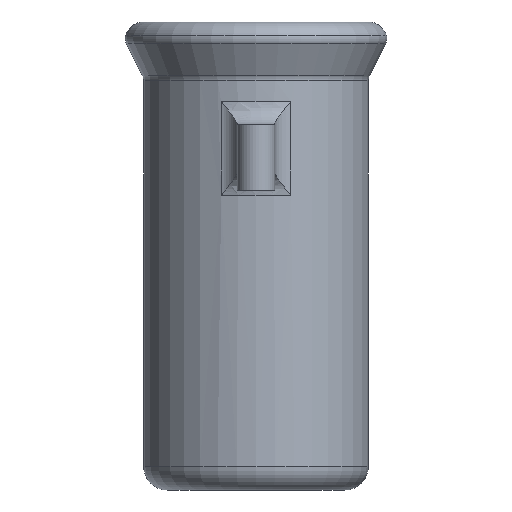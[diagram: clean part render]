
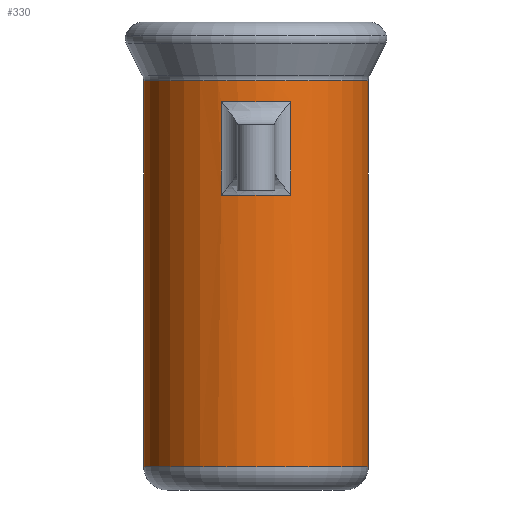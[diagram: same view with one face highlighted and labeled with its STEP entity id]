
A CAD part, front view. The second image highlights one B-rep face of the part: STEP entity #330.
In plain terms, the highlighted cylindrical face has radius 15.24 mm (diameter 30.48 mm), a partial arc.
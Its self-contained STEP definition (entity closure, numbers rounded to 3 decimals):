
#3 = EDGE_LOOP ( 'NONE', ( #1440, #1247, #1269, #567 ) ) ;
#60 = AXIS2_PLACEMENT_3D ( 'NONE', #1375, #1349, #1344 ) ;
#120 = FACE_OUTER_BOUND ( 'NONE', #3, .T. ) ;
#125 = LINE ( 'NONE', #1165, #603 ) ;
#192 = EDGE_CURVE ( 'NONE', #564, #1615, #839, .T. ) ;
#237 = CARTESIAN_POINT ( 'NONE',  ( 4.73, -14.488, 52.705 ) ) ;
#330 = ADVANCED_FACE ( 'NONE', ( #120, #961 ), #1234, .T. ) ;
#337 = DIRECTION ( 'NONE',  ( 1., 0., 0. ) ) ;
#349 = VECTOR ( 'NONE', #1202, 1000. ) ;
#352 = DIRECTION ( 'NONE',  ( 0., 0., 1. ) ) ;
#359 = CARTESIAN_POINT ( 'NONE',  ( 0., 0., 52.705 ) ) ;
#370 = CARTESIAN_POINT ( 'NONE',  ( -15.24, 0., 3.175 ) ) ;
#423 = VERTEX_POINT ( 'NONE', #1650 ) ;
#430 = VECTOR ( 'NONE', #542, 1000. ) ;
#456 = EDGE_CURVE ( 'NONE', #564, #423, #1716, .T. ) ;
#457 = ORIENTED_EDGE ( 'NONE', *, *, #522, .T. ) ;
#471 = EDGE_CURVE ( 'NONE', #1615, #534, #598, .T. ) ;
#475 = LINE ( 'NONE', #640, #430 ) ;
#498 = CARTESIAN_POINT ( 'NONE',  ( -4.73, -14.488, 40.005 ) ) ;
#500 = EDGE_CURVE ( 'NONE', #534, #423, #1430, .T. ) ;
#505 = EDGE_CURVE ( 'NONE', #1567, #708, #1121, .T. ) ;
#511 = DIRECTION ( 'NONE',  ( 1., 0., 0. ) ) ;
#514 = EDGE_CURVE ( 'NONE', #708, #1564, #475, .T. ) ;
#517 = EDGE_CURVE ( 'NONE', #1564, #570, #1556, .T. ) ;
#522 = EDGE_CURVE ( 'NONE', #570, #1567, #125, .T. ) ;
#525 = DIRECTION ( 'NONE',  ( 0., 0., -1. ) ) ;
#532 = CARTESIAN_POINT ( 'NONE',  ( 0., 0., 40.005 ) ) ;
#534 = VERTEX_POINT ( 'NONE', #370 ) ;
#542 = DIRECTION ( 'NONE',  ( 0., 0., 1. ) ) ;
#546 = DIRECTION ( 'NONE',  ( 1., 0., 0. ) ) ;
#553 = DIRECTION ( 'NONE',  ( 0., 0., 1. ) ) ;
#564 = VERTEX_POINT ( 'NONE', #1172 ) ;
#567 = ORIENTED_EDGE ( 'NONE', *, *, #500, .T. ) ;
#570 = VERTEX_POINT ( 'NONE', #237 ) ;
#598 = LINE ( 'NONE', #894, #349 ) ;
#603 = VECTOR ( 'NONE', #633, 1000. ) ;
#622 = CARTESIAN_POINT ( 'NONE',  ( 0., 0., 3.175 ) ) ;
#633 = DIRECTION ( 'NONE',  ( 0., 0., -1. ) ) ;
#640 = CARTESIAN_POINT ( 'NONE',  ( -4.73, -14.488, 63.5 ) ) ;
#708 = VERTEX_POINT ( 'NONE', #498 ) ;
#839 = CIRCLE ( 'NONE', #60, 15.24 ) ;
#894 = CARTESIAN_POINT ( 'NONE',  ( -15.24, 0., 63.5 ) ) ;
#961 = FACE_BOUND ( 'NONE', #1152, .T. ) ;
#1070 = VECTOR ( 'NONE', #1720, 1000. ) ;
#1121 = CIRCLE ( 'NONE', #1304, 15.24 ) ;
#1152 = EDGE_LOOP ( 'NONE', ( #1319, #1461, #1498, #457 ) ) ;
#1165 = CARTESIAN_POINT ( 'NONE',  ( 4.73, -14.488, 63.5 ) ) ;
#1172 = CARTESIAN_POINT ( 'NONE',  ( 15.24, 0., 55.52 ) ) ;
#1202 = DIRECTION ( 'NONE',  ( 0., 0., -1. ) ) ;
#1234 = CYLINDRICAL_SURFACE ( 'NONE', #1702, 15.24 ) ;
#1247 = ORIENTED_EDGE ( 'NONE', *, *, #192, .T. ) ;
#1269 = ORIENTED_EDGE ( 'NONE', *, *, #471, .T. ) ;
#1291 = AXIS2_PLACEMENT_3D ( 'NONE', #359, #352, #337 ) ;
#1304 = AXIS2_PLACEMENT_3D ( 'NONE', #532, #525, #511 ) ;
#1307 = AXIS2_PLACEMENT_3D ( 'NONE', #622, #553, #546 ) ;
#1319 = ORIENTED_EDGE ( 'NONE', *, *, #505, .T. ) ;
#1344 = DIRECTION ( 'NONE',  ( 1., 0., 0. ) ) ;
#1349 = DIRECTION ( 'NONE',  ( 0., 0., -1. ) ) ;
#1375 = CARTESIAN_POINT ( 'NONE',  ( 0., 0., 55.52 ) ) ;
#1407 = CARTESIAN_POINT ( 'NONE',  ( 4.73, -14.488, 40.005 ) ) ;
#1413 = CARTESIAN_POINT ( 'NONE',  ( -15.24, 0., 55.52 ) ) ;
#1430 = CIRCLE ( 'NONE', #1307, 15.24 ) ;
#1440 = ORIENTED_EDGE ( 'NONE', *, *, #456, .F. ) ;
#1451 = CARTESIAN_POINT ( 'NONE',  ( -4.73, -14.488, 52.705 ) ) ;
#1461 = ORIENTED_EDGE ( 'NONE', *, *, #514, .T. ) ;
#1498 = ORIENTED_EDGE ( 'NONE', *, *, #517, .T. ) ;
#1552 = CARTESIAN_POINT ( 'NONE',  ( 0., 0., 63.5 ) ) ;
#1556 = CIRCLE ( 'NONE', #1291, 15.24 ) ;
#1557 = DIRECTION ( 'NONE',  ( 0., 0., -1. ) ) ;
#1564 = VERTEX_POINT ( 'NONE', #1451 ) ;
#1567 = VERTEX_POINT ( 'NONE', #1407 ) ;
#1615 = VERTEX_POINT ( 'NONE', #1413 ) ;
#1650 = CARTESIAN_POINT ( 'NONE',  ( 15.24, 0., 3.175 ) ) ;
#1700 = CARTESIAN_POINT ( 'NONE',  ( 15.24, 0., 63.5 ) ) ;
#1702 = AXIS2_PLACEMENT_3D ( 'NONE', #1552, #1557, #1704 ) ;
#1704 = DIRECTION ( 'NONE',  ( -1., 0., 0. ) ) ;
#1716 = LINE ( 'NONE', #1700, #1070 ) ;
#1720 = DIRECTION ( 'NONE',  ( 0., 0., -1. ) ) ;
